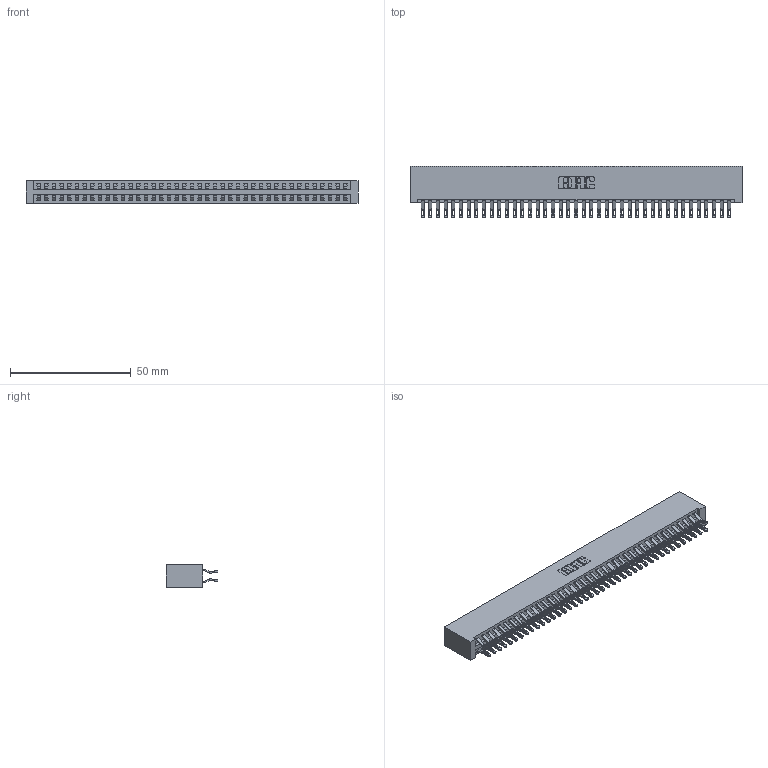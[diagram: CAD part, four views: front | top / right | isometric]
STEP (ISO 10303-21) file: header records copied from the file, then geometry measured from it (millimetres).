
FILE_DESCRIPTION (( 'STEP AP203' ), '1' );
FILE_NAME ('396-082-555-201.STEP', '2019-10-30T23:34:28', ( '' ), ( '' ), 'SwSTEP 2.0', 'SolidWorks 2016', '' );
FILE_SCHEMA (( 'CONFIG_CONTROL_DESIGN' ));
Length unit declared in the file: inch
Products named in the file (3): 346 Part_No Mounting Lugs; 396-082-555-201; 345-292-001_555 Tail
Assembly tree (83 placements, depth 2):
  396-082-555-201
    346 Part_No Mounting Lugs
    345-292-001_555 Tail  x82
Bounding box: 137.41 x 21.46 x 9.4 mm (x, y, z)
Volume: 14202.9 mm3; surface area: 20518.2 mm2
Topology: 83 solids, 83 shells, 4870 faces, 15311 edges, 10206 vertices
Faces by surface type: plane 2778, cylinder 2092
Entity records: 26941 total; most frequent: CARTESIAN_POINT 4474, ORIENTED_EDGE 4378, DIRECTION 3957, EDGE_CURVE 2189, VECTOR 1881, LINE 1881, VERTEX_POINT 1458, AXIS2_PLACEMENT_3D 1038
